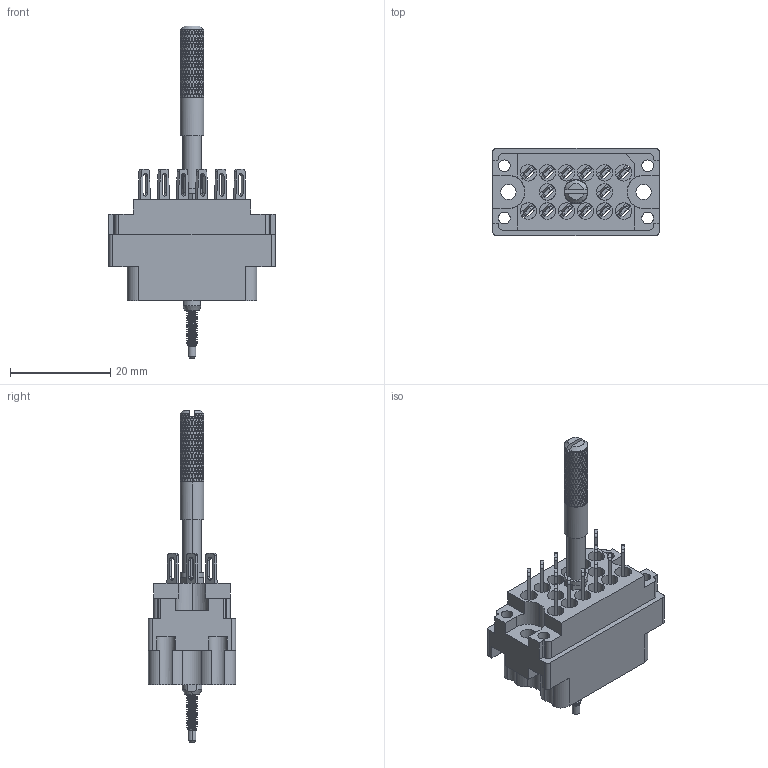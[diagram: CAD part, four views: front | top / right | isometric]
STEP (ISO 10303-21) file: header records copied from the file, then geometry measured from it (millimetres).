
FILE_DESCRIPTION (( 'STEP AP203' ), '1' );
FILE_NAME ('519-014-500-305.STEP', '2020-03-02T20:00:42', ( '' ), ( '' ), 'SwSTEP 2.0', 'SolidWorks 2016', '' );
FILE_SCHEMA (( 'CONFIG_CONTROL_DESIGN' ));
Length unit declared in the file: inch
Products named in the file (9): 516-250-020-111; 519 Plug Insulator_014; 516-253-025-100; 516-252-022-102; 516-292-001_500 Contact; 516-251-025-100; 519-014-500-305; Actuating Screw Assy 020; 516-250-021-102_519
Assembly tree (21 placements, depth 3):
  519-014-500-305
    519 Plug Insulator_014
    516-292-001_500 Contact  x14
    Actuating Screw Assy 020
      516-251-025-100
      516-250-021-102_519
      516-250-020-111
      516-253-025-100
      516-252-022-102
Bounding box: 33.32 x 17.42 x 66.29 mm (x, y, z)
Volume: 6230.5 mm3; surface area: 9941.6 mm2
Topology: 20 solids, 20 shells, 4236 faces, 10082 edges, 5900 vertices
Faces by surface type: bspline 2106, cylinder 1103, plane 1007, cone 20
Entity records: 178295 total; most frequent: CARTESIAN_POINT 128591, ORIENTED_EDGE 14444, EDGE_CURVE 7222, DIRECTION 4956, VERTEX_POINT 4002, EDGE_LOOP 3316, FACE_OUTER_BOUND 3248, ADVANCED_FACE 3248
